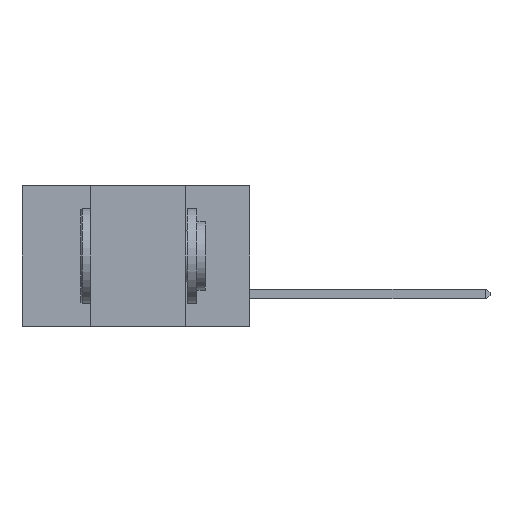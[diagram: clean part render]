
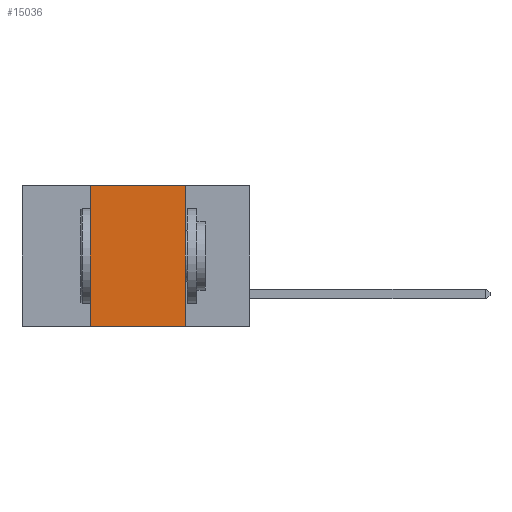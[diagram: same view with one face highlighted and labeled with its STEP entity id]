
A CAD part, left-side view. The second image highlights one B-rep face of the part: STEP entity #15036.
In plain terms, the highlighted planar face has unit normal (-1, 0, 0).
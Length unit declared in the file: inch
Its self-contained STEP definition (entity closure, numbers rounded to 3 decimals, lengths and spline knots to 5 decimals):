
#270 = ORIENTED_EDGE ( 'NONE', *, *, #6842, .F. ) ;
#638 = FACE_OUTER_BOUND ( 'NONE', #12300, .T. ) ;
#3716 = CARTESIAN_POINT ( 'NONE',  ( 0., 0.17, -0.37 ) ) ;
#4316 = EDGE_CURVE ( 'NONE', #16207, #9695, #16403, .T. ) ;
#4376 = LINE ( 'NONE', #19658, #20458 ) ;
#4770 = VECTOR ( 'NONE', #16565, 39.37008 ) ;
#5294 = CARTESIAN_POINT ( 'NONE',  ( 0., 0.42, 0. ) ) ;
#6057 = PLANE ( 'NONE',  #15046 ) ;
#6842 = EDGE_CURVE ( 'NONE', #16207, #11528, #8525, .T. ) ;
#7552 = DIRECTION ( 'NONE',  ( 0., 0., -1. ) ) ;
#7704 = DIRECTION ( 'NONE',  ( 1., 0., 0. ) ) ;
#8525 = LINE ( 'NONE', #18378, #20280 ) ;
#9241 = ORIENTED_EDGE ( 'NONE', *, *, #4316, .T. ) ;
#9695 = VERTEX_POINT ( 'NONE', #3716 ) ;
#10865 = CARTESIAN_POINT ( 'NONE',  ( 0., 0.6, 0. ) ) ;
#11528 = VERTEX_POINT ( 'NONE', #5294 ) ;
#12158 = DIRECTION ( 'NONE',  ( 0., -1., 0. ) ) ;
#12300 = EDGE_LOOP ( 'NONE', ( #20009, #17020, #270, #9241 ) ) ;
#12384 = EDGE_CURVE ( 'NONE', #13257, #9695, #17894, .T. ) ;
#13257 = VERTEX_POINT ( 'NONE', #18328 ) ;
#13825 = CARTESIAN_POINT ( 'NONE',  ( 0., 0.17, 0. ) ) ;
#13872 = VECTOR ( 'NONE', #7552, 39.37008 ) ;
#14569 = CARTESIAN_POINT ( 'NONE',  ( 0., 0.42, -0.37 ) ) ;
#15036 = ADVANCED_FACE ( 'NONE', ( #638 ), #6057, .F. ) ;
#15046 = AXIS2_PLACEMENT_3D ( 'NONE', #10865, #7704, #18512 ) ;
#16207 = VERTEX_POINT ( 'NONE', #14569 ) ;
#16403 = LINE ( 'NONE', #16583, #4770 ) ;
#16565 = DIRECTION ( 'NONE',  ( 0., -1., 0. ) ) ;
#16583 = CARTESIAN_POINT ( 'NONE',  ( 0., 0.6, -0.37 ) ) ;
#17020 = ORIENTED_EDGE ( 'NONE', *, *, #17587, .F. ) ;
#17587 = EDGE_CURVE ( 'NONE', #11528, #13257, #4376, .T. ) ;
#17894 = LINE ( 'NONE', #13825, #13872 ) ;
#18328 = CARTESIAN_POINT ( 'NONE',  ( 0., 0.17, 0. ) ) ;
#18378 = CARTESIAN_POINT ( 'NONE',  ( 0., 0.42, 0. ) ) ;
#18512 = DIRECTION ( 'NONE',  ( 0., 0., -1. ) ) ;
#19658 = CARTESIAN_POINT ( 'NONE',  ( 0., 0.6, 0. ) ) ;
#19863 = DIRECTION ( 'NONE',  ( 0., 0., 1. ) ) ;
#20009 = ORIENTED_EDGE ( 'NONE', *, *, #12384, .F. ) ;
#20280 = VECTOR ( 'NONE', #19863, 39.37008 ) ;
#20458 = VECTOR ( 'NONE', #12158, 39.37008 ) ;
